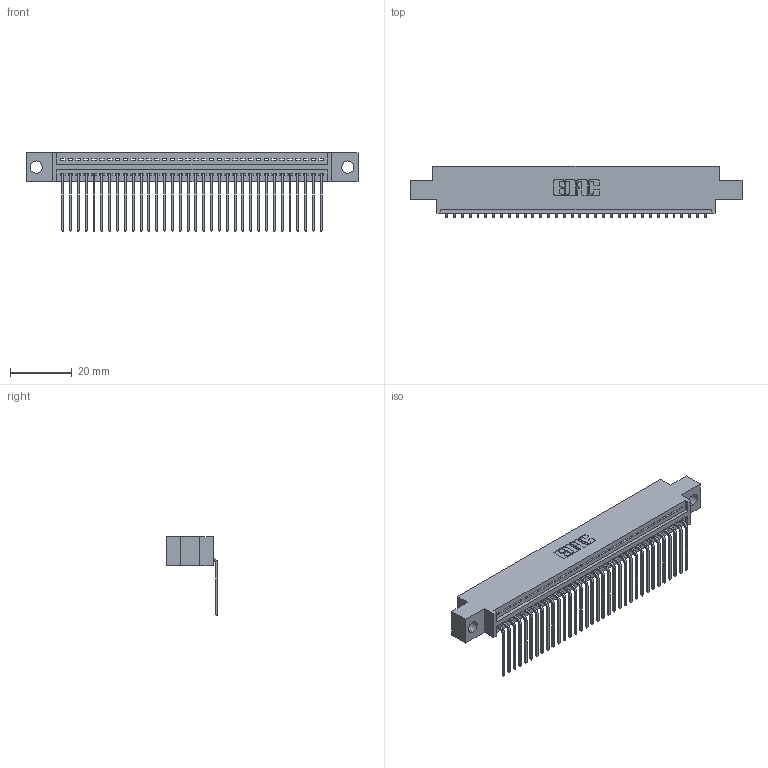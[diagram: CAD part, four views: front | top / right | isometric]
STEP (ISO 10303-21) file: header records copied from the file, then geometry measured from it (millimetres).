
FILE_DESCRIPTION (( 'STEP AP203' ), '1' );
FILE_NAME ('395-034-559-604.STEP', '2021-05-31T14:51:20', ( '' ), ( '' ), 'SwSTEP 2.0', 'SolidWorks 2020', '' );
FILE_SCHEMA (( 'CONFIG_CONTROL_DESIGN' ));
Length unit declared in the file: inch
Products named in the file (3): 345 Part_0.170 Offset - 0.156 Dia-TI; 345-292-001_558 559 Tail - 1; 395-034-559-604
Assembly tree (35 placements, depth 2):
  395-034-559-604
    345 Part_0.170 Offset - 0.156 Dia-TI
    345-292-001_558 559 Tail - 1  x34
Bounding box: 107.57 x 16.75 x 25.53 mm (x, y, z)
Volume: 10045.4 mm3; surface area: 13875.4 mm2
Topology: 35 solids, 35 shells, 2184 faces, 6577 edges, 4338 vertices
Faces by surface type: plane 1526, cylinder 658
Entity records: 27301 total; most frequent: CARTESIAN_POINT 4740, ORIENTED_EDGE 4706, DIRECTION 4149, EDGE_CURVE 2353, VECTOR 2085, LINE 2085, VERTEX_POINT 1566, AXIS2_PLACEMENT_3D 1032
